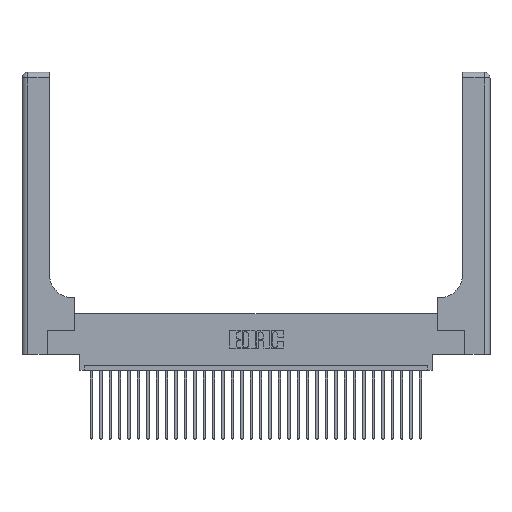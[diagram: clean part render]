
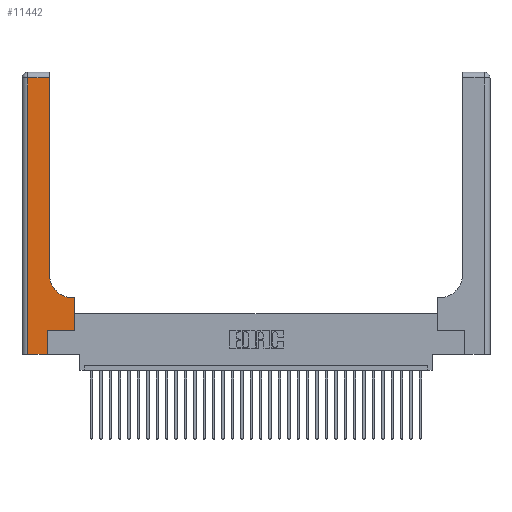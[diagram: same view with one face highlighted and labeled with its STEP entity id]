
A CAD part, top view. The second image highlights one B-rep face of the part: STEP entity #11442.
In plain terms, the highlighted planar face has unit normal (0, 0, 1).
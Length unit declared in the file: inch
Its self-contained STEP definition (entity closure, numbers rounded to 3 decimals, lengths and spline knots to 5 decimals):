
#110 = VERTEX_POINT ( 'NONE', #15595 ) ;
#552 = DIRECTION ( 'NONE',  ( 0., 1., 0. ) ) ;
#1185 = CARTESIAN_POINT ( 'NONE',  ( 0.2915, 0.6, 0.37 ) ) ;
#1931 = DIRECTION ( 'NONE',  ( 0., 0., -1. ) ) ;
#1963 = ORIENTED_EDGE ( 'NONE', *, *, #30510, .T. ) ;
#2146 = DIRECTION ( 'NONE',  ( 0., -1., 0. ) ) ;
#2518 = LINE ( 'NONE', #29509, #32584 ) ;
#3228 = VECTOR ( 'NONE', #25921, 39.37008 ) ;
#3239 = VECTOR ( 'NONE', #10134, 39.37008 ) ;
#3619 = EDGE_CURVE ( 'NONE', #28053, #22451, #12109, .T. ) ;
#3685 = VERTEX_POINT ( 'NONE', #22568 ) ;
#3960 = DIRECTION ( 'NONE',  ( 1., 0., 0. ) ) ;
#4303 = CARTESIAN_POINT ( 'NONE',  ( 0., 3., 0.37 ) ) ;
#5399 = CARTESIAN_POINT ( 'NONE',  ( 0., 0., 0.37 ) ) ;
#6648 = ORIENTED_EDGE ( 'NONE', *, *, #3619, .T. ) ;
#7501 = ORIENTED_EDGE ( 'NONE', *, *, #13360, .T. ) ;
#7927 = ORIENTED_EDGE ( 'NONE', *, *, #25802, .T. ) ;
#8347 = CARTESIAN_POINT ( 'NONE',  ( 0., 2.94, 0.37 ) ) ;
#8387 = FACE_OUTER_BOUND ( 'NONE', #24494, .T. ) ;
#8711 = VERTEX_POINT ( 'NONE', #29310 ) ;
#9286 = VECTOR ( 'NONE', #16144, 39.37008 ) ;
#9443 = CARTESIAN_POINT ( 'NONE',  ( 0.5585, 0.25, 0.37 ) ) ;
#9512 = DIRECTION ( 'NONE',  ( 0., 0., -1. ) ) ;
#9846 = DIRECTION ( 'NONE',  ( -1., 0., 0. ) ) ;
#10134 = DIRECTION ( 'NONE',  ( 0., 1., 0. ) ) ;
#10440 = AXIS2_PLACEMENT_3D ( 'NONE', #24062, #1931, #3960 ) ;
#11160 = ORIENTED_EDGE ( 'NONE', *, *, #30555, .T. ) ;
#11442 = ADVANCED_FACE ( 'NONE', ( #8387 ), #22200, .F. ) ;
#11567 = VERTEX_POINT ( 'NONE', #9443 ) ;
#12109 = LINE ( 'NONE', #17785, #3239 ) ;
#12593 = LINE ( 'NONE', #8347, #17849 ) ;
#12854 = LINE ( 'NONE', #21616, #20526 ) ;
#13360 = EDGE_CURVE ( 'NONE', #11567, #8711, #12854, .T. ) ;
#13829 = DIRECTION ( 'NONE',  ( 0., 1., 0. ) ) ;
#13912 = EDGE_CURVE ( 'NONE', #8711, #20090, #24910, .T. ) ;
#14952 = DIRECTION ( 'NONE',  ( 1., 0., 0. ) ) ;
#15595 = CARTESIAN_POINT ( 'NONE',  ( 0.06, 2.94, 0.37 ) ) ;
#15671 = ORIENTED_EDGE ( 'NONE', *, *, #17916, .T. ) ;
#16144 = DIRECTION ( 'NONE',  ( -1., 0., 0. ) ) ;
#16445 = CARTESIAN_POINT ( 'NONE',  ( 0.2915, 0.85, 0.37 ) ) ;
#17422 = CARTESIAN_POINT ( 'NONE',  ( 0.269, 0.25, 0.37 ) ) ;
#17457 = VECTOR ( 'NONE', #552, 39.37008 ) ;
#17785 = CARTESIAN_POINT ( 'NONE',  ( 0.2915, 3., 0.37 ) ) ;
#17849 = VECTOR ( 'NONE', #31198, 39.37008 ) ;
#17916 = EDGE_CURVE ( 'NONE', #110, #3685, #2518, .T. ) ;
#20090 = VERTEX_POINT ( 'NONE', #26506 ) ;
#20231 = CARTESIAN_POINT ( 'NONE',  ( 0.269, 0.25, 0.37 ) ) ;
#20339 = AXIS2_PLACEMENT_3D ( 'NONE', #4303, #9512, #9846 ) ;
#20344 = ORIENTED_EDGE ( 'NONE', *, *, #30197, .T. ) ;
#20526 = VECTOR ( 'NONE', #13829, 39.37008 ) ;
#20625 = VERTEX_POINT ( 'NONE', #25639 ) ;
#21509 = LINE ( 'NONE', #17422, #33045 ) ;
#21616 = CARTESIAN_POINT ( 'NONE',  ( 0.5585, 0.25, 0.37 ) ) ;
#22097 = ORIENTED_EDGE ( 'NONE', *, *, #31455, .T. ) ;
#22200 = PLANE ( 'NONE',  #20339 ) ;
#22265 = CARTESIAN_POINT ( 'NONE',  ( 0.2915, 2.94, 0.37 ) ) ;
#22451 = VERTEX_POINT ( 'NONE', #22265 ) ;
#22568 = CARTESIAN_POINT ( 'NONE',  ( 0.06, 0., 0.37 ) ) ;
#24062 = CARTESIAN_POINT ( 'NONE',  ( 0.5415, 0.85, 0.37 ) ) ;
#24494 = EDGE_LOOP ( 'NONE', ( #6648, #11160, #15671, #7927, #1963, #20344, #7501, #25628, #22097 ) ) ;
#24910 = LINE ( 'NONE', #1185, #9286 ) ;
#25628 = ORIENTED_EDGE ( 'NONE', *, *, #13912, .T. ) ;
#25639 = CARTESIAN_POINT ( 'NONE',  ( 0.269, 0., 0.37 ) ) ;
#25802 = EDGE_CURVE ( 'NONE', #3685, #20625, #28515, .T. ) ;
#25921 = DIRECTION ( 'NONE',  ( 1., 0., 0. ) ) ;
#26506 = CARTESIAN_POINT ( 'NONE',  ( 0.5415, 0.6, 0.37 ) ) ;
#26618 = LINE ( 'NONE', #31541, #17457 ) ;
#27912 = VERTEX_POINT ( 'NONE', #20231 ) ;
#28053 = VERTEX_POINT ( 'NONE', #16445 ) ;
#28515 = LINE ( 'NONE', #5399, #3228 ) ;
#28950 = CIRCLE ( 'NONE', #10440, 0.25 ) ;
#29310 = CARTESIAN_POINT ( 'NONE',  ( 0.5585, 0.6, 0.37 ) ) ;
#29509 = CARTESIAN_POINT ( 'NONE',  ( 0.06, 3., 0.37 ) ) ;
#30197 = EDGE_CURVE ( 'NONE', #27912, #11567, #21509, .T. ) ;
#30510 = EDGE_CURVE ( 'NONE', #20625, #27912, #26618, .T. ) ;
#30555 = EDGE_CURVE ( 'NONE', #22451, #110, #12593, .T. ) ;
#31198 = DIRECTION ( 'NONE',  ( -1., 0., 0. ) ) ;
#31455 = EDGE_CURVE ( 'NONE', #20090, #28053, #28950, .T. ) ;
#31541 = CARTESIAN_POINT ( 'NONE',  ( 0.269, 0., 0.37 ) ) ;
#32584 = VECTOR ( 'NONE', #2146, 39.37008 ) ;
#33045 = VECTOR ( 'NONE', #14952, 39.37008 ) ;
